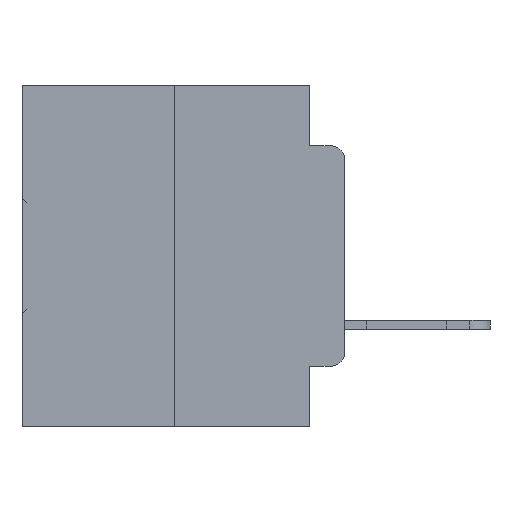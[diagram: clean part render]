
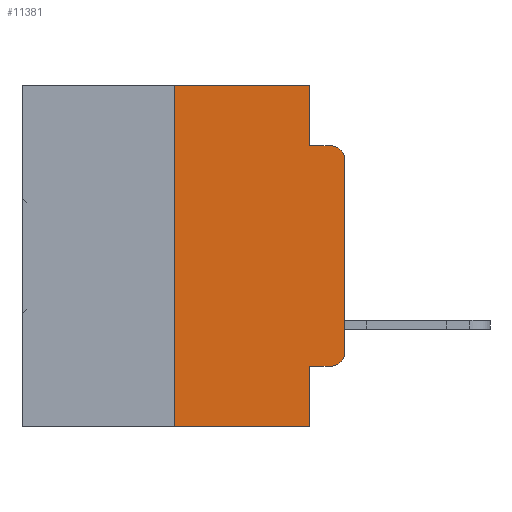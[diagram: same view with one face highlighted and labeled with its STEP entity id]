
A CAD part, left-side view. The second image highlights one B-rep face of the part: STEP entity #11381.
In plain terms, the highlighted planar face has unit normal (-1, 0, 0).
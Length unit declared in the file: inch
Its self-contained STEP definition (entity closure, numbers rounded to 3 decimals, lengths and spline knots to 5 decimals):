
#555 = CARTESIAN_POINT ( 'NONE',  ( 0., 0.051, 0. ) ) ;
#1022 = EDGE_CURVE ( 'NONE', #12992, #21163, #24520, .T. ) ;
#1820 = DIRECTION ( 'NONE',  ( 0., 0., 1. ) ) ;
#2085 = LINE ( 'NONE', #20206, #33057 ) ;
#2984 = VERTEX_POINT ( 'NONE', #5096 ) ;
#3130 = ORIENTED_EDGE ( 'NONE', *, *, #4253, .F. ) ;
#3200 = VERTEX_POINT ( 'NONE', #8838 ) ;
#4253 = EDGE_CURVE ( 'NONE', #12405, #2984, #19175, .T. ) ;
#4305 = EDGE_CURVE ( 'NONE', #3200, #12405, #11070, .T. ) ;
#4536 = ORIENTED_EDGE ( 'NONE', *, *, #1022, .T. ) ;
#4564 = VECTOR ( 'NONE', #19779, 39.37008 ) ;
#5096 = CARTESIAN_POINT ( 'NONE',  ( 0., 0.02, -0.0885 ) ) ;
#5176 = VERTEX_POINT ( 'NONE', #26302 ) ;
#5195 = DIRECTION ( 'NONE',  ( 0., 0., -1. ) ) ;
#5311 = DIRECTION ( 'NONE',  ( 0., -1., 0. ) ) ;
#5352 = CARTESIAN_POINT ( 'NONE',  ( 0., 0.051, -0.4115 ) ) ;
#5730 = ORIENTED_EDGE ( 'NONE', *, *, #5782, .F. ) ;
#5782 = EDGE_CURVE ( 'NONE', #8003, #5176, #2085, .T. ) ;
#6202 = AXIS2_PLACEMENT_3D ( 'NONE', #31103, #16145, #33393 ) ;
#6591 = EDGE_CURVE ( 'NONE', #21821, #2984, #24080, .T. ) ;
#7214 = CARTESIAN_POINT ( 'NONE',  ( 0., 0.02, -0.3915 ) ) ;
#7907 = LINE ( 'NONE', #24028, #33399 ) ;
#8003 = VERTEX_POINT ( 'NONE', #31204 ) ;
#8838 = CARTESIAN_POINT ( 'NONE',  ( 0., 0.051, 0. ) ) ;
#10018 = DIRECTION ( 'NONE',  ( 0., 0., -1. ) ) ;
#10578 = EDGE_CURVE ( 'NONE', #12992, #27793, #17239, .T. ) ;
#10932 = DIRECTION ( 'NONE',  ( 0., -1., 0. ) ) ;
#11070 = LINE ( 'NONE', #555, #16572 ) ;
#11367 = VECTOR ( 'NONE', #5311, 39.37008 ) ;
#11381 = ADVANCED_FACE ( 'NONE', ( #16704 ), #18875, .F. ) ;
#12393 = VECTOR ( 'NONE', #10932, 39.37008 ) ;
#12405 = VERTEX_POINT ( 'NONE', #16617 ) ;
#12615 = VECTOR ( 'NONE', #1820, 39.37008 ) ;
#12752 = EDGE_LOOP ( 'NONE', ( #13031, #33380, #3130, #13097, #24257, #5730, #16877, #26885, #4536, #33430 ) ) ;
#12992 = VERTEX_POINT ( 'NONE', #5352 ) ;
#13031 = ORIENTED_EDGE ( 'NONE', *, *, #32534, .T. ) ;
#13069 = CIRCLE ( 'NONE', #13381, 0.02 ) ;
#13097 = ORIENTED_EDGE ( 'NONE', *, *, #4305, .F. ) ;
#13381 = AXIS2_PLACEMENT_3D ( 'NONE', #7214, #25704, #10018 ) ;
#13806 = EDGE_CURVE ( 'NONE', #21163, #29502, #13069, .T. ) ;
#14095 = LINE ( 'NONE', #16267, #12393 ) ;
#15533 = CARTESIAN_POINT ( 'NONE',  ( 0., 0.051, -0.5 ) ) ;
#15557 = CARTESIAN_POINT ( 'NONE',  ( 0., 0.02, -0.4115 ) ) ;
#16145 = DIRECTION ( 'NONE',  ( -1., 0., 0. ) ) ;
#16267 = CARTESIAN_POINT ( 'NONE',  ( 0., 0.473, -0.5 ) ) ;
#16572 = VECTOR ( 'NONE', #27112, 39.37008 ) ;
#16617 = CARTESIAN_POINT ( 'NONE',  ( 0., 0.051, -0.0885 ) ) ;
#16704 = FACE_OUTER_BOUND ( 'NONE', #12752, .T. ) ;
#16877 = ORIENTED_EDGE ( 'NONE', *, *, #18826, .T. ) ;
#17239 = LINE ( 'NONE', #28442, #23311 ) ;
#18826 = EDGE_CURVE ( 'NONE', #8003, #27793, #14095, .T. ) ;
#18875 = PLANE ( 'NONE',  #30484 ) ;
#19175 = LINE ( 'NONE', #27615, #4564 ) ;
#19479 = DIRECTION ( 'NONE',  ( 0., 0., 1. ) ) ;
#19779 = DIRECTION ( 'NONE',  ( 0., -1., 0. ) ) ;
#20206 = CARTESIAN_POINT ( 'NONE',  ( 0., 0.25, 0. ) ) ;
#21163 = VERTEX_POINT ( 'NONE', #15557 ) ;
#21525 = DIRECTION ( 'NONE',  ( 1., 0., 0. ) ) ;
#21821 = VERTEX_POINT ( 'NONE', #30634 ) ;
#22198 = CARTESIAN_POINT ( 'NONE',  ( 0., 0., -0.3915 ) ) ;
#22609 = CARTESIAN_POINT ( 'NONE',  ( 0., 0.051, -0.4115 ) ) ;
#23311 = VECTOR ( 'NONE', #30826, 39.37008 ) ;
#24028 = CARTESIAN_POINT ( 'NONE',  ( 0., 0.473, 0. ) ) ;
#24080 = CIRCLE ( 'NONE', #6202, 0.02 ) ;
#24257 = ORIENTED_EDGE ( 'NONE', *, *, #31586, .F. ) ;
#24520 = LINE ( 'NONE', #22609, #11367 ) ;
#25704 = DIRECTION ( 'NONE',  ( -1., 0., 0. ) ) ;
#26302 = CARTESIAN_POINT ( 'NONE',  ( 0., 0.25, 0. ) ) ;
#26399 = LINE ( 'NONE', #30577, #12615 ) ;
#26459 = DIRECTION ( 'NONE',  ( 0., -1., 0. ) ) ;
#26885 = ORIENTED_EDGE ( 'NONE', *, *, #10578, .F. ) ;
#27112 = DIRECTION ( 'NONE',  ( 0., 0., -1. ) ) ;
#27615 = CARTESIAN_POINT ( 'NONE',  ( 0., 0.051, -0.0885 ) ) ;
#27793 = VERTEX_POINT ( 'NONE', #15533 ) ;
#28442 = CARTESIAN_POINT ( 'NONE',  ( 0., 0.051, 0. ) ) ;
#29502 = VERTEX_POINT ( 'NONE', #22198 ) ;
#30484 = AXIS2_PLACEMENT_3D ( 'NONE', #31056, #21525, #5195 ) ;
#30577 = CARTESIAN_POINT ( 'NONE',  ( 0., 0., 0. ) ) ;
#30634 = CARTESIAN_POINT ( 'NONE',  ( 0., 0., -0.1085 ) ) ;
#30826 = DIRECTION ( 'NONE',  ( 0., 0., -1. ) ) ;
#31056 = CARTESIAN_POINT ( 'NONE',  ( 0., 0.473, 0. ) ) ;
#31103 = CARTESIAN_POINT ( 'NONE',  ( 0., 0.02, -0.1085 ) ) ;
#31204 = CARTESIAN_POINT ( 'NONE',  ( 0., 0.25, -0.5 ) ) ;
#31586 = EDGE_CURVE ( 'NONE', #5176, #3200, #7907, .T. ) ;
#32534 = EDGE_CURVE ( 'NONE', #29502, #21821, #26399, .T. ) ;
#33057 = VECTOR ( 'NONE', #19479, 39.37008 ) ;
#33380 = ORIENTED_EDGE ( 'NONE', *, *, #6591, .T. ) ;
#33393 = DIRECTION ( 'NONE',  ( 0., 0., -1. ) ) ;
#33399 = VECTOR ( 'NONE', #26459, 39.37008 ) ;
#33430 = ORIENTED_EDGE ( 'NONE', *, *, #13806, .T. ) ;
